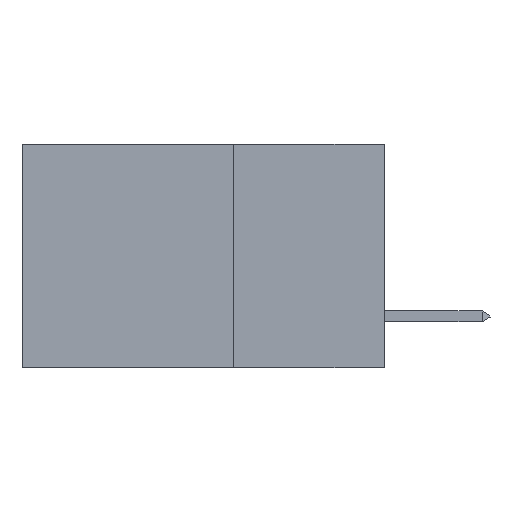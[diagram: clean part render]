
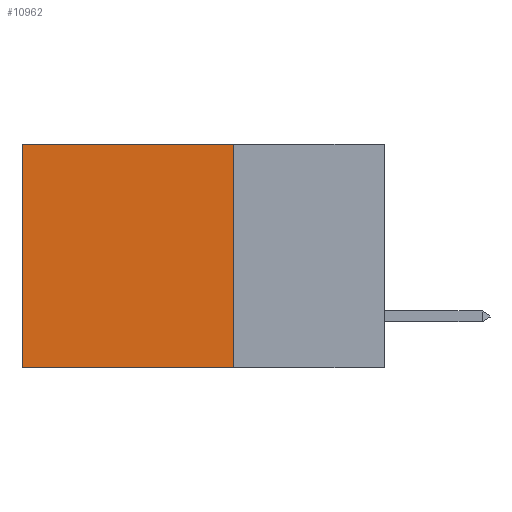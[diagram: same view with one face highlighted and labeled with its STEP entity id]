
A CAD part, left-side view. The second image highlights one B-rep face of the part: STEP entity #10962.
In plain terms, the highlighted planar face has unit normal (-1, 0, 0).
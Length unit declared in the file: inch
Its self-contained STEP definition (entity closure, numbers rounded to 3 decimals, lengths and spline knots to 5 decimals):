
#256 = LINE ( 'NONE', #22387, #20487 ) ;
#616 = ORIENTED_EDGE ( 'NONE', *, *, #12878, .T. ) ;
#1160 = VECTOR ( 'NONE', #37953, 39.37008 ) ;
#1497 = VECTOR ( 'NONE', #21302, 39.37008 ) ;
#2083 = EDGE_CURVE ( 'NONE', #4736, #10207, #12959, .T. ) ;
#3237 = PLANE ( 'NONE',  #37833 ) ;
#3663 = VERTEX_POINT ( 'NONE', #22626 ) ;
#4736 = VERTEX_POINT ( 'NONE', #10508 ) ;
#4909 = VECTOR ( 'NONE', #8208, 39.37008 ) ;
#8208 = DIRECTION ( 'NONE',  ( 0., 1., 0. ) ) ;
#8801 = CARTESIAN_POINT ( 'NONE',  ( 0.2875, 0.6, -0.37 ) ) ;
#8838 = ORIENTED_EDGE ( 'NONE', *, *, #26454, .T. ) ;
#10207 = VERTEX_POINT ( 'NONE', #8801 ) ;
#10356 = EDGE_LOOP ( 'NONE', ( #8838, #39684, #32919, #616 ) ) ;
#10508 = CARTESIAN_POINT ( 'NONE',  ( 0.2875, 0.25, -0.37 ) ) ;
#10962 = ADVANCED_FACE ( 'NONE', ( #35982 ), #3237, .F. ) ;
#12878 = EDGE_CURVE ( 'NONE', #16041, #3663, #256, .T. ) ;
#12959 = LINE ( 'NONE', #17595, #4909 ) ;
#13704 = CARTESIAN_POINT ( 'NONE',  ( 0.2875, 0.6, 0. ) ) ;
#16041 = VERTEX_POINT ( 'NONE', #25272 ) ;
#16061 = LINE ( 'NONE', #13704, #1160 ) ;
#16343 = DIRECTION ( 'NONE',  ( 0., 1., 0. ) ) ;
#17595 = CARTESIAN_POINT ( 'NONE',  ( 0.2875, 0.25, -0.37 ) ) ;
#20487 = VECTOR ( 'NONE', #16343, 39.37008 ) ;
#21302 = DIRECTION ( 'NONE',  ( 0., 0., -1. ) ) ;
#22387 = CARTESIAN_POINT ( 'NONE',  ( 0.2875, 0.25, 0. ) ) ;
#22626 = CARTESIAN_POINT ( 'NONE',  ( 0.2875, 0.6, 0. ) ) ;
#24722 = CARTESIAN_POINT ( 'NONE',  ( 0.2875, 0.25, 0. ) ) ;
#25272 = CARTESIAN_POINT ( 'NONE',  ( 0.2875, 0.25, 0. ) ) ;
#25924 = DIRECTION ( 'NONE',  ( 0., 0., -1. ) ) ;
#26454 = EDGE_CURVE ( 'NONE', #3663, #10207, #16061, .T. ) ;
#27810 = DIRECTION ( 'NONE',  ( 1., 0., 0. ) ) ;
#28518 = EDGE_CURVE ( 'NONE', #16041, #4736, #37469, .T. ) ;
#32919 = ORIENTED_EDGE ( 'NONE', *, *, #28518, .F. ) ;
#33337 = CARTESIAN_POINT ( 'NONE',  ( 0.2875, 0.25, 0. ) ) ;
#35982 = FACE_OUTER_BOUND ( 'NONE', #10356, .T. ) ;
#37469 = LINE ( 'NONE', #33337, #1497 ) ;
#37833 = AXIS2_PLACEMENT_3D ( 'NONE', #24722, #27810, #25924 ) ;
#37953 = DIRECTION ( 'NONE',  ( 0., 0., -1. ) ) ;
#39684 = ORIENTED_EDGE ( 'NONE', *, *, #2083, .F. ) ;
